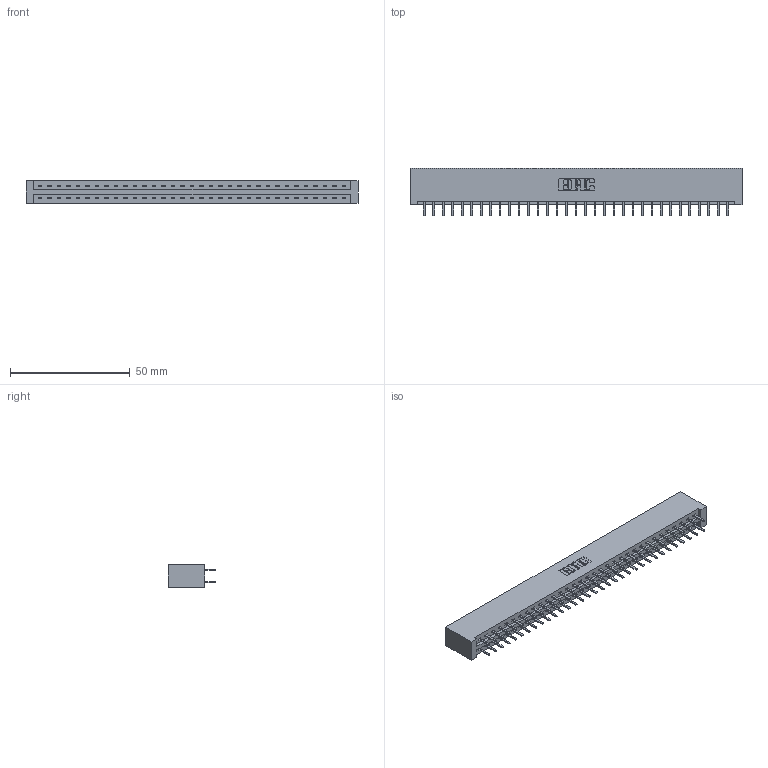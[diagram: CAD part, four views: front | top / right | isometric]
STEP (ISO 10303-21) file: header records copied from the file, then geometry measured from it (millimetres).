
FILE_DESCRIPTION (( 'STEP AP203' ), '1' );
FILE_NAME ('387-066-520-201.STEP', '2018-09-21T08:58:36', ( '' ), ( '' ), 'SwSTEP 2.0', 'SolidWorks 2016', '' );
FILE_SCHEMA (( 'CONFIG_CONTROL_DESIGN' ));
Length unit declared in the file: inch
Products named in the file (3): 337 Part_No Mounting Lugs; 345-292-001_345-293-120; 387-066-520-201
Assembly tree (67 placements, depth 2):
  387-066-520-201
    337 Part_No Mounting Lugs
    345-292-001_345-293-120  x66
Bounding box: 138.63 x 20.02 x 9.4 mm (x, y, z)
Volume: 15222.2 mm3; surface area: 17094.6 mm2
Topology: 67 solids, 67 shells, 3934 faces, 11441 edges, 7450 vertices
Faces by surface type: plane 2706, cylinder 1228
Entity records: 26587 total; most frequent: CARTESIAN_POINT 4498, ORIENTED_EDGE 4422, DIRECTION 3823, EDGE_CURVE 2211, VECTOR 2087, LINE 2087, VERTEX_POINT 1470, AXIS2_PLACEMENT_3D 868
